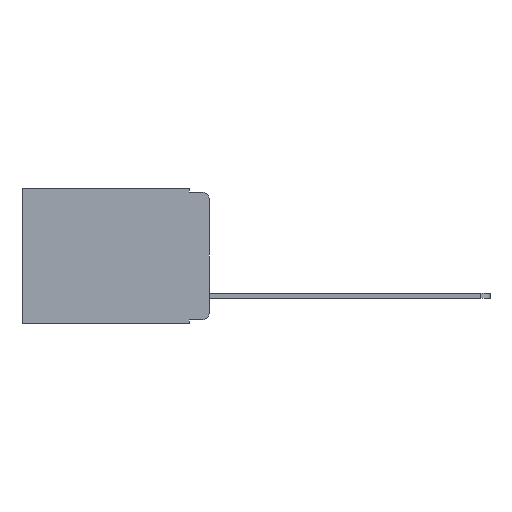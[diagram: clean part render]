
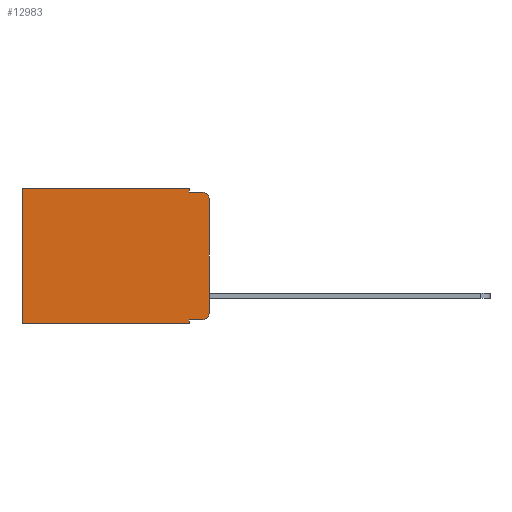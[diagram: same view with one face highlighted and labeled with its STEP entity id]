
A CAD part, left-side view. The second image highlights one B-rep face of the part: STEP entity #12983.
In plain terms, the highlighted planar face has unit normal (-1, 0, 0).
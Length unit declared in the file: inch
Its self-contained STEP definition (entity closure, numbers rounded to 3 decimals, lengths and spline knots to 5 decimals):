
#90 = CARTESIAN_POINT ( 'NONE',  ( 0.298, 0.02, -0.03 ) ) ;
#205 = DIRECTION ( 'NONE',  ( 1., 0., 0. ) ) ;
#267 = LINE ( 'NONE', #5156, #3419 ) ;
#384 = CARTESIAN_POINT ( 'NONE',  ( 0.298, 0., -0.03 ) ) ;
#409 = EDGE_CURVE ( 'NONE', #14163, #18215, #7730, .T. ) ;
#439 = EDGE_CURVE ( 'NONE', #14163, #8475, #11134, .T. ) ;
#442 = EDGE_CURVE ( 'NONE', #4461, #8475, #17048, .T. ) ;
#469 = EDGE_CURVE ( 'NONE', #1273, #4461, #6286, .T. ) ;
#470 = EDGE_CURVE ( 'NONE', #11520, #762, #10225, .T. ) ;
#478 = EDGE_CURVE ( 'NONE', #12355, #3303, #1849, .T. ) ;
#496 = EDGE_CURVE ( 'NONE', #12355, #1500, #9330, .T. ) ;
#500 = EDGE_CURVE ( 'NONE', #1500, #18215, #15777, .T. ) ;
#657 = ORIENTED_EDGE ( 'NONE', *, *, #478, .F. ) ;
#762 = VERTEX_POINT ( 'NONE', #12463 ) ;
#1185 = ORIENTED_EDGE ( 'NONE', *, *, #409, .F. ) ;
#1273 = VERTEX_POINT ( 'NONE', #16802 ) ;
#1500 = VERTEX_POINT ( 'NONE', #18056 ) ;
#1849 = LINE ( 'NONE', #4499, #12687 ) ;
#2169 = DIRECTION ( 'NONE',  ( 0., 1., 0. ) ) ;
#2308 = CARTESIAN_POINT ( 'NONE',  ( 0.298, 0.051, -0.333 ) ) ;
#2743 = FACE_OUTER_BOUND ( 'NONE', #11948, .T. ) ;
#3303 = VERTEX_POINT ( 'NONE', #9389 ) ;
#3389 = ORIENTED_EDGE ( 'NONE', *, *, #500, .T. ) ;
#3419 = VECTOR ( 'NONE', #2169, 39.37008 ) ;
#3533 = DIRECTION ( 'NONE',  ( 0., 0., -1. ) ) ;
#3794 = DIRECTION ( 'NONE',  ( 0., 0., -1. ) ) ;
#3925 = AXIS2_PLACEMENT_3D ( 'NONE', #90, #17276, #3794 ) ;
#4461 = VERTEX_POINT ( 'NONE', #14889 ) ;
#4499 = CARTESIAN_POINT ( 'NONE',  ( 0.298, 0.051, 0. ) ) ;
#4765 = CARTESIAN_POINT ( 'NONE',  ( 0.298, 0.051, 0. ) ) ;
#4872 = VECTOR ( 'NONE', #12316, 39.37008 ) ;
#4909 = ORIENTED_EDGE ( 'NONE', *, *, #7408, .T. ) ;
#5156 = CARTESIAN_POINT ( 'NONE',  ( 0.298, 0., -0.343 ) ) ;
#5810 = VECTOR ( 'NONE', #3533, 39.37008 ) ;
#6017 = DIRECTION ( 'NONE',  ( 0., 0., -1. ) ) ;
#6286 = LINE ( 'NONE', #4765, #16638 ) ;
#6853 = CARTESIAN_POINT ( 'NONE',  ( 0.298, 0.02, -0.313 ) ) ;
#7035 = DIRECTION ( 'NONE',  ( 0., 1., 0. ) ) ;
#7408 = EDGE_CURVE ( 'NONE', #1273, #11520, #15704, .T. ) ;
#7730 = LINE ( 'NONE', #15070, #17895 ) ;
#7808 = PLANE ( 'NONE',  #18410 ) ;
#7809 = CARTESIAN_POINT ( 'NONE',  ( 0.298, 0.051, -0.01 ) ) ;
#8283 = DIRECTION ( 'NONE',  ( 0., 0., -1. ) ) ;
#8449 = ORIENTED_EDGE ( 'NONE', *, *, #17457, .F. ) ;
#8475 = VERTEX_POINT ( 'NONE', #13934 ) ;
#8953 = AXIS2_PLACEMENT_3D ( 'NONE', #6853, #16482, #6017 ) ;
#9330 = LINE ( 'NONE', #2308, #4872 ) ;
#9389 = CARTESIAN_POINT ( 'NONE',  ( 0.298, 0.051, -0.343 ) ) ;
#9494 = DIRECTION ( 'NONE',  ( 0., 0., -1. ) ) ;
#9577 = CARTESIAN_POINT ( 'NONE',  ( 0.298, 0.051, -0.333 ) ) ;
#9740 = ORIENTED_EDGE ( 'NONE', *, *, #470, .T. ) ;
#10049 = CARTESIAN_POINT ( 'NONE',  ( 0.298, 0., 0. ) ) ;
#10225 = LINE ( 'NONE', #14376, #5810 ) ;
#10436 = DIRECTION ( 'NONE',  ( 0., 0., -1. ) ) ;
#10583 = ORIENTED_EDGE ( 'NONE', *, *, #469, .F. ) ;
#10727 = DIRECTION ( 'NONE',  ( 0., 0., -1. ) ) ;
#10746 = ORIENTED_EDGE ( 'NONE', *, *, #442, .F. ) ;
#11134 = CIRCLE ( 'NONE', #3925, 0.02 ) ;
#11520 = VERTEX_POINT ( 'NONE', #13566 ) ;
#11741 = VECTOR ( 'NONE', #7035, 39.37008 ) ;
#11948 = EDGE_LOOP ( 'NONE', ( #1185, #14808, #10746, #10583, #4909, #9740, #8449, #657, #16916, #3389 ) ) ;
#12316 = DIRECTION ( 'NONE',  ( 0., -1., 0. ) ) ;
#12355 = VERTEX_POINT ( 'NONE', #9577 ) ;
#12463 = CARTESIAN_POINT ( 'NONE',  ( 0.298, 0.473, -0.343 ) ) ;
#12520 = CARTESIAN_POINT ( 'NONE',  ( 0.298, 0., -0.313 ) ) ;
#12687 = VECTOR ( 'NONE', #8283, 39.37008 ) ;
#12983 = ADVANCED_FACE ( 'NONE', ( #2743 ), #7808, .F. ) ;
#13544 = VECTOR ( 'NONE', #13951, 39.37008 ) ;
#13566 = CARTESIAN_POINT ( 'NONE',  ( 0.298, 0.473, 0. ) ) ;
#13934 = CARTESIAN_POINT ( 'NONE',  ( 0.298, 0.02, -0.01 ) ) ;
#13951 = DIRECTION ( 'NONE',  ( 0., -1., 0. ) ) ;
#14163 = VERTEX_POINT ( 'NONE', #384 ) ;
#14376 = CARTESIAN_POINT ( 'NONE',  ( 0.298, 0.473, 0. ) ) ;
#14808 = ORIENTED_EDGE ( 'NONE', *, *, #439, .T. ) ;
#14889 = CARTESIAN_POINT ( 'NONE',  ( 0.298, 0.051, -0.01 ) ) ;
#15070 = CARTESIAN_POINT ( 'NONE',  ( 0.298, 0., 0. ) ) ;
#15704 = LINE ( 'NONE', #10049, #11741 ) ;
#15777 = CIRCLE ( 'NONE', #8953, 0.02 ) ;
#16482 = DIRECTION ( 'NONE',  ( -1., 0., 0. ) ) ;
#16638 = VECTOR ( 'NONE', #9494, 39.37008 ) ;
#16802 = CARTESIAN_POINT ( 'NONE',  ( 0.298, 0.051, 0. ) ) ;
#16916 = ORIENTED_EDGE ( 'NONE', *, *, #496, .T. ) ;
#17048 = LINE ( 'NONE', #7809, #13544 ) ;
#17276 = DIRECTION ( 'NONE',  ( -1., 0., 0. ) ) ;
#17457 = EDGE_CURVE ( 'NONE', #3303, #762, #267, .T. ) ;
#17482 = CARTESIAN_POINT ( 'NONE',  ( 0.298, 0., 0. ) ) ;
#17895 = VECTOR ( 'NONE', #10436, 39.37008 ) ;
#18056 = CARTESIAN_POINT ( 'NONE',  ( 0.298, 0.02, -0.333 ) ) ;
#18215 = VERTEX_POINT ( 'NONE', #12520 ) ;
#18410 = AXIS2_PLACEMENT_3D ( 'NONE', #17482, #205, #10727 ) ;
